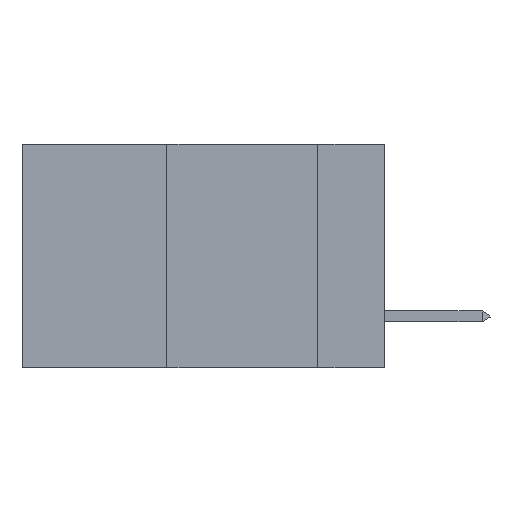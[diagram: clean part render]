
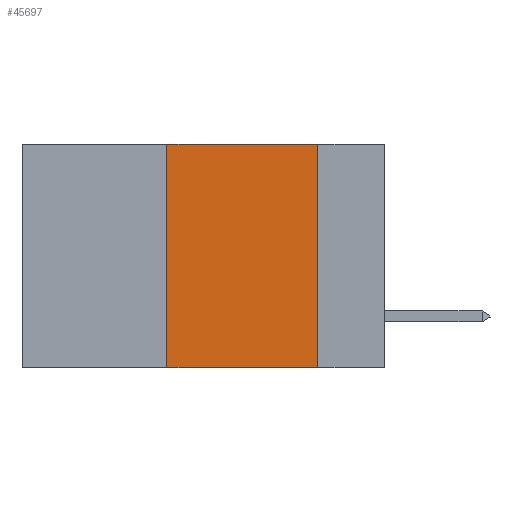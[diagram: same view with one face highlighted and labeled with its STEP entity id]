
A CAD part, left-side view. The second image highlights one B-rep face of the part: STEP entity #45697.
In plain terms, the highlighted planar face has unit normal (-1, 0, 0).
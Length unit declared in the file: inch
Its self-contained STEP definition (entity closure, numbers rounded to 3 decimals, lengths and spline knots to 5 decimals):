
#213 = CARTESIAN_POINT ( 'NONE',  ( 0., 0.36, -0.37 ) ) ;
#2579 = CARTESIAN_POINT ( 'NONE',  ( 0., 0.11, 0. ) ) ;
#3303 = ORIENTED_EDGE ( 'NONE', *, *, #40955, .F. ) ;
#4554 = CARTESIAN_POINT ( 'NONE',  ( 0., 0.36, 0. ) ) ;
#4716 = VERTEX_POINT ( 'NONE', #4554 ) ;
#4903 = ORIENTED_EDGE ( 'NONE', *, *, #8572, .T. ) ;
#6866 = VECTOR ( 'NONE', #22252, 39.37008 ) ;
#8572 = EDGE_CURVE ( 'NONE', #27451, #35786, #27380, .T. ) ;
#10476 = CARTESIAN_POINT ( 'NONE',  ( 0., 0.6, 0. ) ) ;
#11112 = EDGE_LOOP ( 'NONE', ( #15181, #21739, #3303, #4903 ) ) ;
#12036 = DIRECTION ( 'NONE',  ( 0., 0., -1. ) ) ;
#12469 = CARTESIAN_POINT ( 'NONE',  ( 0., 0.11, 0. ) ) ;
#14546 = CARTESIAN_POINT ( 'NONE',  ( 0., 0.6, -0.37 ) ) ;
#15181 = ORIENTED_EDGE ( 'NONE', *, *, #18851, .F. ) ;
#15402 = DIRECTION ( 'NONE',  ( 1., 0., 0. ) ) ;
#18851 = EDGE_CURVE ( 'NONE', #19784, #35786, #21854, .T. ) ;
#19784 = VERTEX_POINT ( 'NONE', #2579 ) ;
#19793 = VECTOR ( 'NONE', #42696, 39.37008 ) ;
#21739 = ORIENTED_EDGE ( 'NONE', *, *, #39560, .F. ) ;
#21854 = LINE ( 'NONE', #12469, #28985 ) ;
#22252 = DIRECTION ( 'NONE',  ( 0., -1., 0. ) ) ;
#23376 = CARTESIAN_POINT ( 'NONE',  ( 0., 0.36, 0. ) ) ;
#26908 = LINE ( 'NONE', #23376, #19793 ) ;
#27380 = LINE ( 'NONE', #14546, #28596 ) ;
#27451 = VERTEX_POINT ( 'NONE', #213 ) ;
#27485 = AXIS2_PLACEMENT_3D ( 'NONE', #45666, #15402, #12036 ) ;
#27724 = DIRECTION ( 'NONE',  ( 0., 0., -1. ) ) ;
#28596 = VECTOR ( 'NONE', #44501, 39.37008 ) ;
#28985 = VECTOR ( 'NONE', #27724, 39.37008 ) ;
#33420 = CARTESIAN_POINT ( 'NONE',  ( 0., 0.11, -0.37 ) ) ;
#34266 = LINE ( 'NONE', #10476, #6866 ) ;
#34506 = PLANE ( 'NONE',  #27485 ) ;
#35786 = VERTEX_POINT ( 'NONE', #33420 ) ;
#39560 = EDGE_CURVE ( 'NONE', #4716, #19784, #34266, .T. ) ;
#40955 = EDGE_CURVE ( 'NONE', #27451, #4716, #26908, .T. ) ;
#42696 = DIRECTION ( 'NONE',  ( 0., 0., 1. ) ) ;
#44501 = DIRECTION ( 'NONE',  ( 0., -1., 0. ) ) ;
#45666 = CARTESIAN_POINT ( 'NONE',  ( 0., 0.6, 0. ) ) ;
#45697 = ADVANCED_FACE ( 'NONE', ( #48751 ), #34506, .F. ) ;
#48751 = FACE_OUTER_BOUND ( 'NONE', #11112, .T. ) ;
